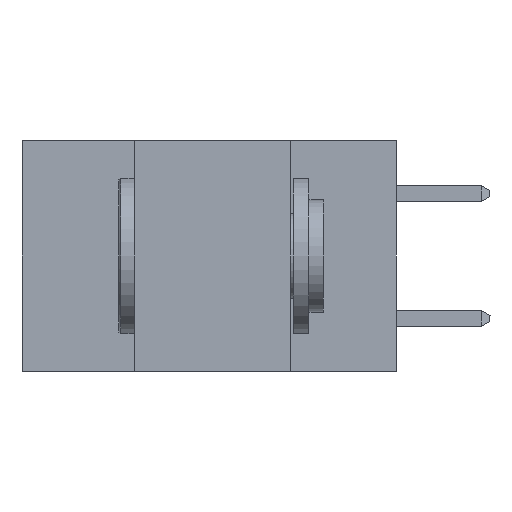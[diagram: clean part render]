
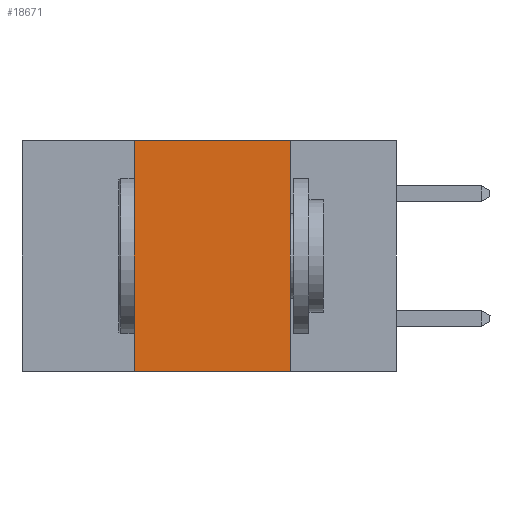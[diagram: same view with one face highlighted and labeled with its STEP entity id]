
A CAD part, left-side view. The second image highlights one B-rep face of the part: STEP entity #18671.
In plain terms, the highlighted planar face has unit normal (-1, 0, 0).
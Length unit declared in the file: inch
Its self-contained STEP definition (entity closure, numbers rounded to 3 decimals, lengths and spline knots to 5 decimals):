
#137 = DIRECTION ( 'NONE',  ( 0., 0., 1. ) ) ;
#613 = ORIENTED_EDGE ( 'NONE', *, *, #12125, .F. ) ;
#704 = CARTESIAN_POINT ( 'NONE',  ( 0., 0.6, -0.37 ) ) ;
#1554 = CARTESIAN_POINT ( 'NONE',  ( 0., 0.6, 0. ) ) ;
#2528 = VECTOR ( 'NONE', #12292, 39.37008 ) ;
#3594 = EDGE_LOOP ( 'NONE', ( #613, #13736, #19865, #7845 ) ) ;
#5051 = LINE ( 'NONE', #29767, #21001 ) ;
#5774 = VERTEX_POINT ( 'NONE', #7598 ) ;
#6330 = LINE ( 'NONE', #704, #31934 ) ;
#7598 = CARTESIAN_POINT ( 'NONE',  ( 0., 0.17, -0.37 ) ) ;
#7845 = ORIENTED_EDGE ( 'NONE', *, *, #12331, .T. ) ;
#9340 = EDGE_CURVE ( 'NONE', #20959, #27949, #17826, .T. ) ;
#9417 = PLANE ( 'NONE',  #17522 ) ;
#12125 = EDGE_CURVE ( 'NONE', #27949, #5774, #24619, .T. ) ;
#12292 = DIRECTION ( 'NONE',  ( 0., 0., -1. ) ) ;
#12331 = EDGE_CURVE ( 'NONE', #27583, #5774, #6330, .T. ) ;
#13736 = ORIENTED_EDGE ( 'NONE', *, *, #9340, .F. ) ;
#17057 = CARTESIAN_POINT ( 'NONE',  ( 0., 0.6, 0. ) ) ;
#17522 = AXIS2_PLACEMENT_3D ( 'NONE', #1554, #31316, #31640 ) ;
#17602 = CARTESIAN_POINT ( 'NONE',  ( 0., 0.42, -0.37 ) ) ;
#17826 = LINE ( 'NONE', #17057, #20948 ) ;
#17943 = CARTESIAN_POINT ( 'NONE',  ( 0., 0.42, 0. ) ) ;
#18075 = FACE_OUTER_BOUND ( 'NONE', #3594, .T. ) ;
#18671 = ADVANCED_FACE ( 'NONE', ( #18075 ), #9417, .F. ) ;
#19865 = ORIENTED_EDGE ( 'NONE', *, *, #20847, .F. ) ;
#20847 = EDGE_CURVE ( 'NONE', #27583, #20959, #5051, .T. ) ;
#20899 = DIRECTION ( 'NONE',  ( 0., -1., 0. ) ) ;
#20948 = VECTOR ( 'NONE', #29528, 39.37008 ) ;
#20959 = VERTEX_POINT ( 'NONE', #17943 ) ;
#21001 = VECTOR ( 'NONE', #137, 39.37008 ) ;
#24619 = LINE ( 'NONE', #29472, #2528 ) ;
#27583 = VERTEX_POINT ( 'NONE', #17602 ) ;
#27949 = VERTEX_POINT ( 'NONE', #30717 ) ;
#29472 = CARTESIAN_POINT ( 'NONE',  ( 0., 0.17, 0. ) ) ;
#29528 = DIRECTION ( 'NONE',  ( 0., -1., 0. ) ) ;
#29767 = CARTESIAN_POINT ( 'NONE',  ( 0., 0.42, 0. ) ) ;
#30717 = CARTESIAN_POINT ( 'NONE',  ( 0., 0.17, 0. ) ) ;
#31316 = DIRECTION ( 'NONE',  ( 1., 0., 0. ) ) ;
#31640 = DIRECTION ( 'NONE',  ( 0., 0., -1. ) ) ;
#31934 = VECTOR ( 'NONE', #20899, 39.37008 ) ;
